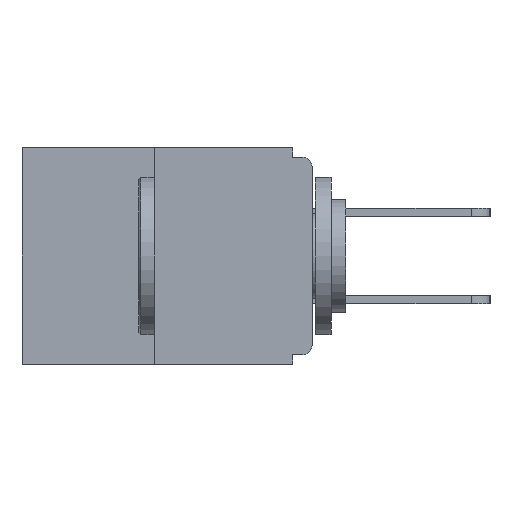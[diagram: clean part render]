
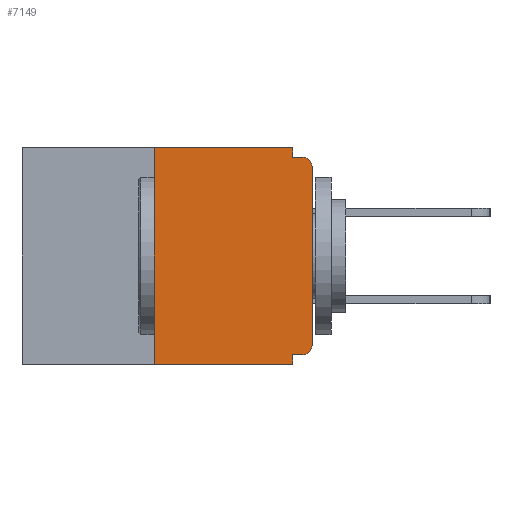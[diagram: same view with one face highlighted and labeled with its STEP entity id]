
A CAD part, left-side view. The second image highlights one B-rep face of the part: STEP entity #7149.
In plain terms, the highlighted planar face has unit normal (-1, 0, 0).
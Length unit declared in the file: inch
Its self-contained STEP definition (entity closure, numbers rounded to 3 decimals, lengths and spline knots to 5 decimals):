
#91 = EDGE_CURVE ( 'NONE', #534, #5262, #4425, .T. ) ;
#157 = VECTOR ( 'NONE', #8378, 39.37008 ) ;
#263 = EDGE_CURVE ( 'NONE', #580, #1946, #12298, .T. ) ;
#273 = ORIENTED_EDGE ( 'NONE', *, *, #13382, .F. ) ;
#332 = CARTESIAN_POINT ( 'NONE',  ( 0., 0.25, 0. ) ) ;
#484 = FACE_OUTER_BOUND ( 'NONE', #5920, .T. ) ;
#534 = VERTEX_POINT ( 'NONE', #6883 ) ;
#580 = VERTEX_POINT ( 'NONE', #737 ) ;
#590 = VERTEX_POINT ( 'NONE', #13640 ) ;
#711 = EDGE_CURVE ( 'NONE', #10802, #13075, #4891, .T. ) ;
#737 = CARTESIAN_POINT ( 'NONE',  ( 0., 0.031, -0.015 ) ) ;
#963 = ORIENTED_EDGE ( 'NONE', *, *, #1026, .F. ) ;
#1026 = EDGE_CURVE ( 'NONE', #4637, #5397, #5432, .T. ) ;
#1028 = ORIENTED_EDGE ( 'NONE', *, *, #91, .T. ) ;
#1073 = CARTESIAN_POINT ( 'NONE',  ( 0., 0., -0.015 ) ) ;
#1141 = LINE ( 'NONE', #8857, #3664 ) ;
#1148 = CARTESIAN_POINT ( 'NONE',  ( 0., 0.031, -0.343 ) ) ;
#1387 = CIRCLE ( 'NONE', #10613, 0.015 ) ;
#1906 = CARTESIAN_POINT ( 'NONE',  ( 0., 0.015, -0.015 ) ) ;
#1946 = VERTEX_POINT ( 'NONE', #1906 ) ;
#2167 = DIRECTION ( 'NONE',  ( 0., -1., 0. ) ) ;
#2258 = CARTESIAN_POINT ( 'NONE',  ( 0., 0.015, -0.03 ) ) ;
#2582 = ORIENTED_EDGE ( 'NONE', *, *, #263, .F. ) ;
#2616 = LINE ( 'NONE', #8862, #11988 ) ;
#2619 = DIRECTION ( 'NONE',  ( 0., 0., -1. ) ) ;
#3275 = EDGE_CURVE ( 'NONE', #7339, #13075, #2616, .T. ) ;
#3664 = VECTOR ( 'NONE', #10090, 39.37008 ) ;
#4184 = LINE ( 'NONE', #7315, #157 ) ;
#4252 = VECTOR ( 'NONE', #6966, 39.37008 ) ;
#4287 = ORIENTED_EDGE ( 'NONE', *, *, #9586, .F. ) ;
#4302 = DIRECTION ( 'NONE',  ( -1., 0., 0. ) ) ;
#4308 = CARTESIAN_POINT ( 'NONE',  ( 0., 0.25, -0.343 ) ) ;
#4362 = ORIENTED_EDGE ( 'NONE', *, *, #3275, .T. ) ;
#4425 = LINE ( 'NONE', #13739, #11780 ) ;
#4637 = VERTEX_POINT ( 'NONE', #332 ) ;
#4722 = CARTESIAN_POINT ( 'NONE',  ( 0., 0.015, -0.313 ) ) ;
#4815 = CARTESIAN_POINT ( 'NONE',  ( 0., 0.46, 0. ) ) ;
#4891 = LINE ( 'NONE', #1148, #10440 ) ;
#5131 = VECTOR ( 'NONE', #13315, 39.37008 ) ;
#5262 = VERTEX_POINT ( 'NONE', #13446 ) ;
#5397 = VERTEX_POINT ( 'NONE', #7348 ) ;
#5432 = LINE ( 'NONE', #9190, #4252 ) ;
#5920 = EDGE_LOOP ( 'NONE', ( #963, #8353, #4362, #13043, #4287, #6560, #1028, #11804, #2582, #273 ) ) ;
#6560 = ORIENTED_EDGE ( 'NONE', *, *, #11626, .T. ) ;
#6883 = CARTESIAN_POINT ( 'NONE',  ( 0., 0., -0.313 ) ) ;
#6966 = DIRECTION ( 'NONE',  ( 0., -1., 0. ) ) ;
#6994 = AXIS2_PLACEMENT_3D ( 'NONE', #4815, #12330, #10405 ) ;
#7149 = ADVANCED_FACE ( 'NONE', ( #484 ), #9316, .F. ) ;
#7315 = CARTESIAN_POINT ( 'NONE',  ( 0., 0.031, 0. ) ) ;
#7339 = VERTEX_POINT ( 'NONE', #4308 ) ;
#7348 = CARTESIAN_POINT ( 'NONE',  ( 0., 0.031, 0. ) ) ;
#7401 = DIRECTION ( 'NONE',  ( 0., 0., 1. ) ) ;
#8294 = EDGE_CURVE ( 'NONE', #7339, #4637, #1141, .T. ) ;
#8353 = ORIENTED_EDGE ( 'NONE', *, *, #8294, .F. ) ;
#8378 = DIRECTION ( 'NONE',  ( 0., 0., -1. ) ) ;
#8857 = CARTESIAN_POINT ( 'NONE',  ( 0., 0.25, 0. ) ) ;
#8862 = CARTESIAN_POINT ( 'NONE',  ( 0., 0.46, -0.343 ) ) ;
#9190 = CARTESIAN_POINT ( 'NONE',  ( 0., 0.46, 0. ) ) ;
#9316 = PLANE ( 'NONE',  #6994 ) ;
#9586 = EDGE_CURVE ( 'NONE', #590, #10802, #11827, .T. ) ;
#9783 = DIRECTION ( 'NONE',  ( 0., 0., -1. ) ) ;
#10090 = DIRECTION ( 'NONE',  ( 0., 0., 1. ) ) ;
#10298 = CIRCLE ( 'NONE', #12670, 0.015 ) ;
#10405 = DIRECTION ( 'NONE',  ( 0., 0., -1. ) ) ;
#10440 = VECTOR ( 'NONE', #11586, 39.37008 ) ;
#10613 = AXIS2_PLACEMENT_3D ( 'NONE', #4722, #12215, #2619 ) ;
#10802 = VERTEX_POINT ( 'NONE', #13888 ) ;
#10888 = EDGE_CURVE ( 'NONE', #5262, #1946, #10298, .T. ) ;
#10910 = CARTESIAN_POINT ( 'NONE',  ( 0., 0., -0.328 ) ) ;
#11586 = DIRECTION ( 'NONE',  ( 0., 0., -1. ) ) ;
#11626 = EDGE_CURVE ( 'NONE', #590, #534, #1387, .T. ) ;
#11780 = VECTOR ( 'NONE', #7401, 39.37008 ) ;
#11804 = ORIENTED_EDGE ( 'NONE', *, *, #10888, .T. ) ;
#11827 = LINE ( 'NONE', #10910, #5131 ) ;
#11988 = VECTOR ( 'NONE', #12052, 39.37008 ) ;
#12052 = DIRECTION ( 'NONE',  ( 0., -1., 0. ) ) ;
#12121 = VECTOR ( 'NONE', #2167, 39.37008 ) ;
#12215 = DIRECTION ( 'NONE',  ( -1., 0., 0. ) ) ;
#12298 = LINE ( 'NONE', #1073, #12121 ) ;
#12330 = DIRECTION ( 'NONE',  ( 1., 0., 0. ) ) ;
#12670 = AXIS2_PLACEMENT_3D ( 'NONE', #2258, #4302, #9783 ) ;
#13043 = ORIENTED_EDGE ( 'NONE', *, *, #711, .F. ) ;
#13075 = VERTEX_POINT ( 'NONE', #13322 ) ;
#13315 = DIRECTION ( 'NONE',  ( 0., 1., 0. ) ) ;
#13322 = CARTESIAN_POINT ( 'NONE',  ( 0., 0.031, -0.343 ) ) ;
#13382 = EDGE_CURVE ( 'NONE', #5397, #580, #4184, .T. ) ;
#13446 = CARTESIAN_POINT ( 'NONE',  ( 0., 0., -0.03 ) ) ;
#13640 = CARTESIAN_POINT ( 'NONE',  ( 0., 0.015, -0.328 ) ) ;
#13739 = CARTESIAN_POINT ( 'NONE',  ( 0., 0., 0. ) ) ;
#13888 = CARTESIAN_POINT ( 'NONE',  ( 0., 0.031, -0.328 ) ) ;
